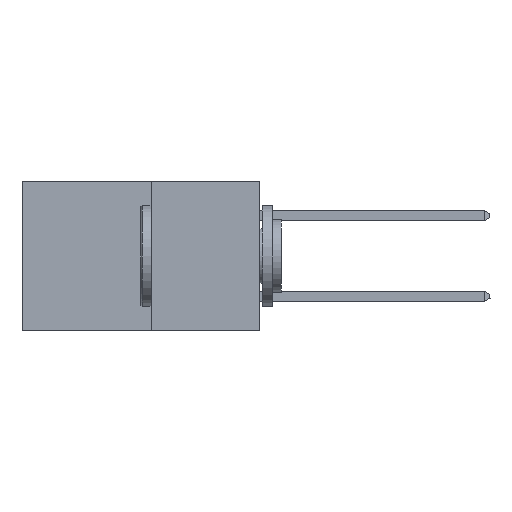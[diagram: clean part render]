
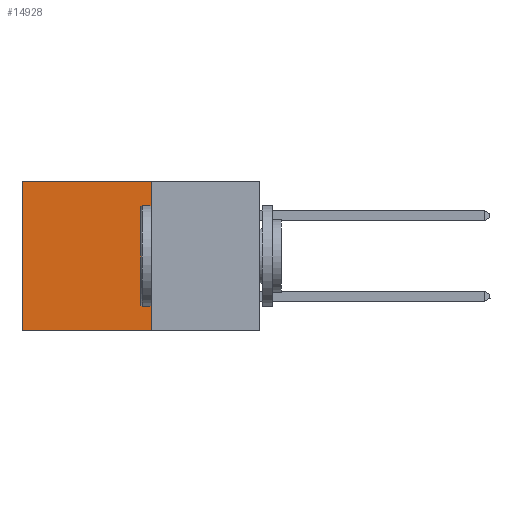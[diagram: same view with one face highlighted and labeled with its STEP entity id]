
A CAD part, left-side view. The second image highlights one B-rep face of the part: STEP entity #14928.
In plain terms, the highlighted planar face has unit normal (-1, 0, 0).
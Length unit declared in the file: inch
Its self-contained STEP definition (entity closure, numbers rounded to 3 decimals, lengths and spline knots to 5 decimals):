
#145 = DIRECTION ( 'NONE',  ( 0., 0., -1. ) ) ;
#259 = CARTESIAN_POINT ( 'NONE',  ( 0.277, 0.59, -0.37 ) ) ;
#2419 = PLANE ( 'NONE',  #10312 ) ;
#3084 = EDGE_LOOP ( 'NONE', ( #17562, #25808, #6575, #24590 ) ) ;
#6575 = ORIENTED_EDGE ( 'NONE', *, *, #17088, .F. ) ;
#6807 = DIRECTION ( 'NONE',  ( 0., 0., -1. ) ) ;
#6984 = CARTESIAN_POINT ( 'NONE',  ( 0.277, 0.27, 0. ) ) ;
#7010 = DIRECTION ( 'NONE',  ( 0., 1., 0. ) ) ;
#7425 = VERTEX_POINT ( 'NONE', #19697 ) ;
#7464 = VERTEX_POINT ( 'NONE', #19403 ) ;
#8501 = EDGE_CURVE ( 'NONE', #23951, #7464, #27475, .T. ) ;
#8987 = EDGE_CURVE ( 'NONE', #7464, #7425, #20499, .T. ) ;
#10312 = AXIS2_PLACEMENT_3D ( 'NONE', #25799, #19498, #6807 ) ;
#12286 = CARTESIAN_POINT ( 'NONE',  ( 0.277, 0.27, -0.37 ) ) ;
#12687 = VECTOR ( 'NONE', #14119, 39.37008 ) ;
#13279 = VERTEX_POINT ( 'NONE', #12286 ) ;
#14119 = DIRECTION ( 'NONE',  ( 0., 1., 0. ) ) ;
#14914 = VECTOR ( 'NONE', #145, 39.37008 ) ;
#14928 = ADVANCED_FACE ( 'NONE', ( #24990 ), #2419, .F. ) ;
#16299 = VECTOR ( 'NONE', #7010, 39.37008 ) ;
#16314 = VECTOR ( 'NONE', #18432, 39.37008 ) ;
#17088 = EDGE_CURVE ( 'NONE', #23951, #13279, #17604, .T. ) ;
#17562 = ORIENTED_EDGE ( 'NONE', *, *, #8987, .T. ) ;
#17604 = LINE ( 'NONE', #24712, #16314 ) ;
#18432 = DIRECTION ( 'NONE',  ( 0., 0., -1. ) ) ;
#19403 = CARTESIAN_POINT ( 'NONE',  ( 0.277, 0.59, 0. ) ) ;
#19498 = DIRECTION ( 'NONE',  ( 1., 0., 0. ) ) ;
#19697 = CARTESIAN_POINT ( 'NONE',  ( 0.277, 0.59, -0.37 ) ) ;
#20499 = LINE ( 'NONE', #259, #14914 ) ;
#20648 = CARTESIAN_POINT ( 'NONE',  ( 0.277, 0.27, 0. ) ) ;
#21529 = EDGE_CURVE ( 'NONE', #13279, #7425, #23906, .T. ) ;
#23906 = LINE ( 'NONE', #26864, #12687 ) ;
#23951 = VERTEX_POINT ( 'NONE', #20648 ) ;
#24590 = ORIENTED_EDGE ( 'NONE', *, *, #8501, .T. ) ;
#24712 = CARTESIAN_POINT ( 'NONE',  ( 0.277, 0.27, -0.37 ) ) ;
#24990 = FACE_OUTER_BOUND ( 'NONE', #3084, .T. ) ;
#25799 = CARTESIAN_POINT ( 'NONE',  ( 0.277, 0.27, -0.37 ) ) ;
#25808 = ORIENTED_EDGE ( 'NONE', *, *, #21529, .F. ) ;
#26864 = CARTESIAN_POINT ( 'NONE',  ( 0.277, 0.27, -0.37 ) ) ;
#27475 = LINE ( 'NONE', #6984, #16299 ) ;
